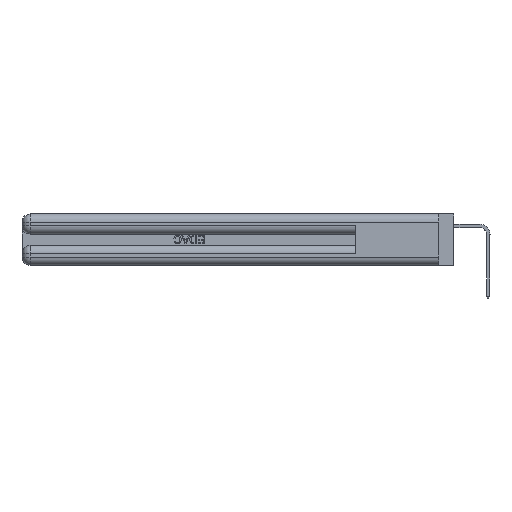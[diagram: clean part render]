
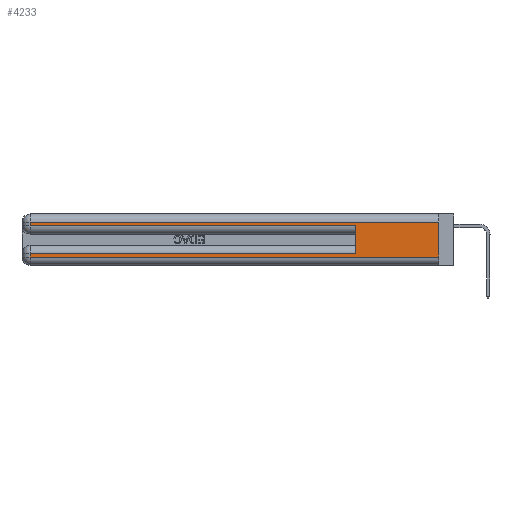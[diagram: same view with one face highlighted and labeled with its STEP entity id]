
A CAD part, left-side view. The second image highlights one B-rep face of the part: STEP entity #4233.
In plain terms, the highlighted planar face has unit normal (-1, 0, 0).
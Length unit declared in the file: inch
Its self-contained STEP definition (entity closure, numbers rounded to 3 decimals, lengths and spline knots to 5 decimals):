
#853 = DIRECTION ( 'NONE',  ( 0., 0., -1. ) ) ;
#1140 = CARTESIAN_POINT ( 'NONE',  ( 0., 2.94, 0.31 ) ) ;
#2354 = DIRECTION ( 'NONE',  ( 0., 1., 0. ) ) ;
#2694 = EDGE_LOOP ( 'NONE', ( #37335, #35937, #36057, #41312, #15738, #40008, #33102, #13207 ) ) ;
#3327 = DIRECTION ( 'NONE',  ( 1., 0., 0. ) ) ;
#4233 = ADVANCED_FACE ( 'NONE', ( #15039 ), #50701, .F. ) ;
#4921 = CARTESIAN_POINT ( 'NONE',  ( 0., 2.94, 0.06 ) ) ;
#4984 = AXIS2_PLACEMENT_3D ( 'NONE', #7132, #3327, #30960 ) ;
#5123 = EDGE_CURVE ( 'NONE', #42675, #44259, #5730, .T. ) ;
#5295 = VERTEX_POINT ( 'NONE', #29318 ) ;
#5730 = LINE ( 'NONE', #24474, #26723 ) ;
#5910 = CARTESIAN_POINT ( 'NONE',  ( 0., 2.94, 0.085 ) ) ;
#6593 = DIRECTION ( 'NONE',  ( 0., -1., 0. ) ) ;
#7132 = CARTESIAN_POINT ( 'NONE',  ( 0., 0., 0.37 ) ) ;
#7827 = EDGE_CURVE ( 'NONE', #11419, #12482, #36009, .T. ) ;
#8508 = DIRECTION ( 'NONE',  ( 0., 0., -1. ) ) ;
#9004 = CARTESIAN_POINT ( 'NONE',  ( 0., 2.94, 0.285 ) ) ;
#10285 = CARTESIAN_POINT ( 'NONE',  ( 0., 0., 0.085 ) ) ;
#11419 = VERTEX_POINT ( 'NONE', #9004 ) ;
#12482 = VERTEX_POINT ( 'NONE', #26798 ) ;
#13207 = ORIENTED_EDGE ( 'NONE', *, *, #42853, .T. ) ;
#13514 = VERTEX_POINT ( 'NONE', #29824 ) ;
#15039 = FACE_OUTER_BOUND ( 'NONE', #2694, .T. ) ;
#15738 = ORIENTED_EDGE ( 'NONE', *, *, #46693, .F. ) ;
#16441 = CARTESIAN_POINT ( 'NONE',  ( 0., 0.6, 0.085 ) ) ;
#18113 = LINE ( 'NONE', #28011, #39181 ) ;
#18793 = DIRECTION ( 'NONE',  ( 0., -1., 0. ) ) ;
#19491 = VECTOR ( 'NONE', #8508, 39.37008 ) ;
#20398 = VERTEX_POINT ( 'NONE', #1140 ) ;
#20530 = VECTOR ( 'NONE', #31095, 39.37008 ) ;
#21596 = LINE ( 'NONE', #10285, #30887 ) ;
#22052 = EDGE_CURVE ( 'NONE', #13514, #5295, #41628, .T. ) ;
#24474 = CARTESIAN_POINT ( 'NONE',  ( 0., 2.94, 0.37 ) ) ;
#25448 = VECTOR ( 'NONE', #6593, 39.37008 ) ;
#26293 = EDGE_CURVE ( 'NONE', #20398, #11419, #30052, .T. ) ;
#26694 = VERTEX_POINT ( 'NONE', #16441 ) ;
#26723 = VECTOR ( 'NONE', #853, 39.37008 ) ;
#26798 = CARTESIAN_POINT ( 'NONE',  ( 0., 0.6, 0.285 ) ) ;
#28011 = CARTESIAN_POINT ( 'NONE',  ( 0., 0.6, 0.145 ) ) ;
#29318 = CARTESIAN_POINT ( 'NONE',  ( 0., 0., 0.06 ) ) ;
#29824 = CARTESIAN_POINT ( 'NONE',  ( 0., 0., 0.31 ) ) ;
#30052 = LINE ( 'NONE', #32004, #19491 ) ;
#30887 = VECTOR ( 'NONE', #2354, 39.37008 ) ;
#30960 = DIRECTION ( 'NONE',  ( 0., 0., -1. ) ) ;
#31095 = DIRECTION ( 'NONE',  ( 0., 0., -1. ) ) ;
#31793 = DIRECTION ( 'NONE',  ( 0., 0., 1. ) ) ;
#32004 = CARTESIAN_POINT ( 'NONE',  ( 0., 2.94, 0.37 ) ) ;
#33102 = ORIENTED_EDGE ( 'NONE', *, *, #5123, .T. ) ;
#35937 = ORIENTED_EDGE ( 'NONE', *, *, #47091, .T. ) ;
#36009 = LINE ( 'NONE', #46023, #25448 ) ;
#36057 = ORIENTED_EDGE ( 'NONE', *, *, #26293, .T. ) ;
#37039 = CARTESIAN_POINT ( 'NONE',  ( 0., 0., 0.31 ) ) ;
#37335 = ORIENTED_EDGE ( 'NONE', *, *, #22052, .F. ) ;
#38377 = CARTESIAN_POINT ( 'NONE',  ( 0., 0., 0.06 ) ) ;
#39065 = CARTESIAN_POINT ( 'NONE',  ( 0., 0., 0.37 ) ) ;
#39181 = VECTOR ( 'NONE', #31793, 39.37008 ) ;
#40008 = ORIENTED_EDGE ( 'NONE', *, *, #48431, .T. ) ;
#41027 = DIRECTION ( 'NONE',  ( 0., 1., 0. ) ) ;
#41312 = ORIENTED_EDGE ( 'NONE', *, *, #7827, .T. ) ;
#41628 = LINE ( 'NONE', #39065, #20530 ) ;
#42675 = VERTEX_POINT ( 'NONE', #5910 ) ;
#42822 = VECTOR ( 'NONE', #41027, 39.37008 ) ;
#42853 = EDGE_CURVE ( 'NONE', #44259, #5295, #45942, .T. ) ;
#43436 = VECTOR ( 'NONE', #18793, 39.37008 ) ;
#44078 = LINE ( 'NONE', #37039, #42822 ) ;
#44259 = VERTEX_POINT ( 'NONE', #4921 ) ;
#45942 = LINE ( 'NONE', #38377, #43436 ) ;
#46023 = CARTESIAN_POINT ( 'NONE',  ( 0., 0., 0.285 ) ) ;
#46693 = EDGE_CURVE ( 'NONE', #26694, #12482, #18113, .T. ) ;
#47091 = EDGE_CURVE ( 'NONE', #13514, #20398, #44078, .T. ) ;
#48431 = EDGE_CURVE ( 'NONE', #26694, #42675, #21596, .T. ) ;
#50701 = PLANE ( 'NONE',  #4984 ) ;
